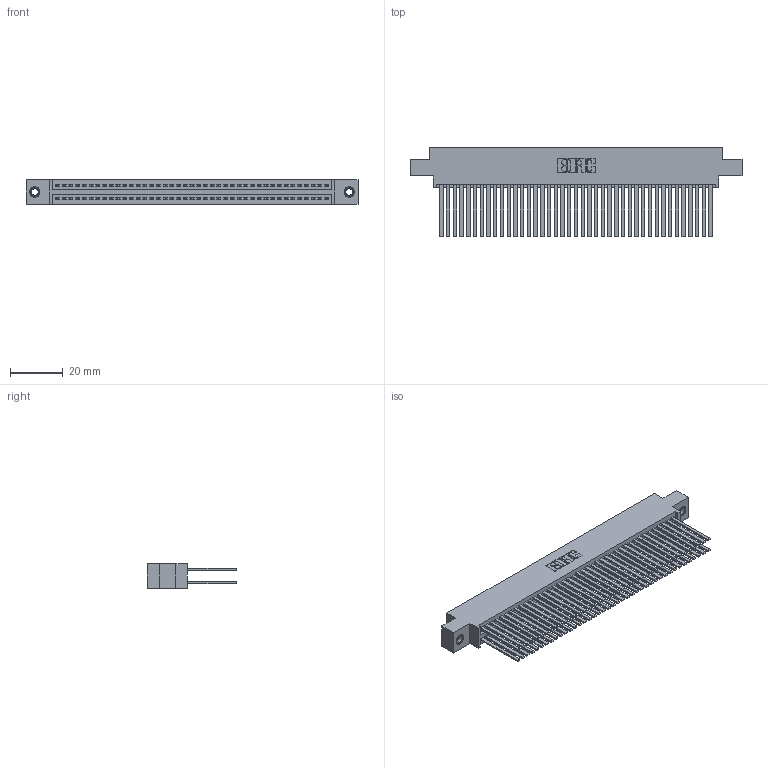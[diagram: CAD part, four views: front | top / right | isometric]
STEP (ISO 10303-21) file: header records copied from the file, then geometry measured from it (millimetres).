
FILE_DESCRIPTION (( 'STEP AP203' ), '1' );
FILE_NAME ('395-082-544-807.STEP', '2019-10-25T07:03:43', ( '' ), ( '' ), 'SwSTEP 2.0', 'SolidWorks 2016', '' );
FILE_SCHEMA (( 'CONFIG_CONTROL_DESIGN' ));
Length unit declared in the file: inch
Products named in the file (4): 345 Part_0.170 Offset - 0.156 Dia-TI; 345-292-001_345-293-144; 345-250-001_345-250-005-103; 395-082-544-807
Assembly tree (85 placements, depth 2):
  395-082-544-807
    345 Part_0.170 Offset - 0.156 Dia-TI
    345-292-001_345-293-144  x82
    345-250-001_345-250-005-103  x2
Bounding box: 125.35 x 33.96 x 9.4 mm (x, y, z)
Volume: 13189.8 mm3; surface area: 23017.8 mm2
Topology: 85 solids, 85 shells, 3798 faces, 11231 edges, 7370 vertices
Faces by surface type: plane 2494, cylinder 1288, cone 12, torus 4
Entity records: 33438 total; most frequent: CARTESIAN_POINT 5587, ORIENTED_EDGE 5514, DIRECTION 4951, EDGE_CURVE 2757, LINE 2445, VECTOR 2445, VERTEX_POINT 1832, AXIS2_PLACEMENT_3D 1253
